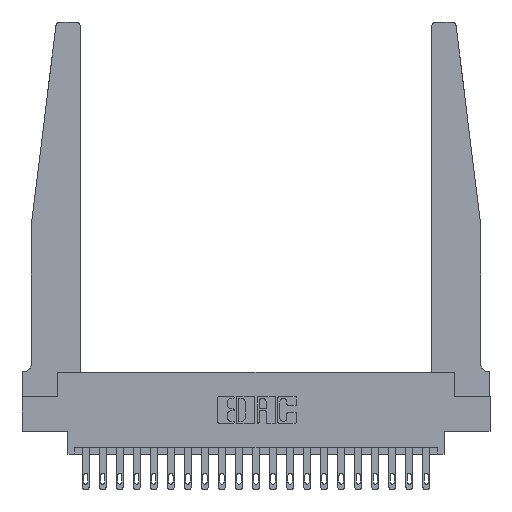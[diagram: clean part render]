
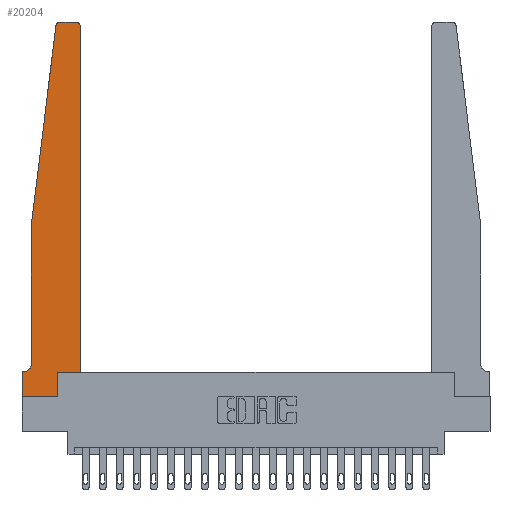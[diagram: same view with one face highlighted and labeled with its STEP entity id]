
A CAD part, top view. The second image highlights one B-rep face of the part: STEP entity #20204.
In plain terms, the highlighted planar face has unit normal (0, 0, 1).
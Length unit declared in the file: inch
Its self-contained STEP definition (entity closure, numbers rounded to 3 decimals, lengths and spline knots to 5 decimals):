
#179 = CARTESIAN_POINT ( 'NONE',  ( 0., 0., 0.37 ) ) ;
#238 = EDGE_CURVE ( 'NONE', #3607, #6068, #4222, .T. ) ;
#278 = CARTESIAN_POINT ( 'NONE',  ( 0.2605, 0.18, 0.37 ) ) ;
#815 = LINE ( 'NONE', #18837, #13661 ) ;
#883 = VECTOR ( 'NONE', #14829, 39.37008 ) ;
#1017 = VECTOR ( 'NONE', #2385, 39.37008 ) ;
#1247 = ORIENTED_EDGE ( 'NONE', *, *, #8335, .T. ) ;
#1311 = CIRCLE ( 'NONE', #14009, 0.05 ) ;
#1351 = LINE ( 'NONE', #5009, #883 ) ;
#1422 = DIRECTION ( 'NONE',  ( 0., 1., 0. ) ) ;
#2039 = ORIENTED_EDGE ( 'NONE', *, *, #21047, .T. ) ;
#2239 = DIRECTION ( 'NONE',  ( 0., 0., -1. ) ) ;
#2385 = DIRECTION ( 'NONE',  ( -1., 0., 0. ) ) ;
#2437 = CARTESIAN_POINT ( 'NONE',  ( 0., 0.1875, 0.37 ) ) ;
#2565 = LINE ( 'NONE', #7774, #5900 ) ;
#2585 = ORIENTED_EDGE ( 'NONE', *, *, #16935, .T. ) ;
#2627 = VECTOR ( 'NONE', #11093, 39.37008 ) ;
#2864 = EDGE_CURVE ( 'NONE', #7976, #3607, #16387, .T. ) ;
#3026 = AXIS2_PLACEMENT_3D ( 'NONE', #9695, #9591, #19854 ) ;
#3241 = CARTESIAN_POINT ( 'NONE',  ( 0.2605, 0., 0.37 ) ) ;
#3318 = CARTESIAN_POINT ( 'NONE',  ( 0.065, 0.2375, 0.37 ) ) ;
#3509 = DIRECTION ( 'NONE',  ( 0., -1., 0. ) ) ;
#3607 = VERTEX_POINT ( 'NONE', #5739 ) ;
#3970 = VERTEX_POINT ( 'NONE', #9327 ) ;
#4222 = LINE ( 'NONE', #18913, #10289 ) ;
#4361 = CARTESIAN_POINT ( 'NONE',  ( 0.27653, 2.75, 0.37 ) ) ;
#4724 = VECTOR ( 'NONE', #3509, 39.37008 ) ;
#5009 = CARTESIAN_POINT ( 'NONE',  ( 0., 0., 0.37 ) ) ;
#5739 = CARTESIAN_POINT ( 'NONE',  ( 0.065, 1.25, 0.37 ) ) ;
#5900 = VECTOR ( 'NONE', #14396, 39.37008 ) ;
#6068 = VERTEX_POINT ( 'NONE', #3318 ) ;
#6510 = AXIS2_PLACEMENT_3D ( 'NONE', #6581, #12978, #16644 ) ;
#6581 = CARTESIAN_POINT ( 'NONE',  ( 0.395, 2.72, 0.37 ) ) ;
#6965 = ORIENTED_EDGE ( 'NONE', *, *, #20962, .T. ) ;
#6979 = LINE ( 'NONE', #13712, #1017 ) ;
#7196 = ORIENTED_EDGE ( 'NONE', *, *, #17585, .T. ) ;
#7213 = DIRECTION ( 'NONE',  ( 0., -1., 0. ) ) ;
#7774 = CARTESIAN_POINT ( 'NONE',  ( 0.2605, 0.18, 0.37 ) ) ;
#7828 = CARTESIAN_POINT ( 'NONE',  ( 0.425, 0.18, 0.37 ) ) ;
#7976 = VERTEX_POINT ( 'NONE', #10484 ) ;
#8082 = CARTESIAN_POINT ( 'NONE',  ( 0.425, 0.18, 0.37 ) ) ;
#8148 = FACE_OUTER_BOUND ( 'NONE', #20293, .T. ) ;
#8335 = EDGE_CURVE ( 'NONE', #17377, #21127, #19267, .T. ) ;
#8602 = CARTESIAN_POINT ( 'NONE',  ( 0.27653, 2.72, 0.37 ) ) ;
#8771 = DIRECTION ( 'NONE',  ( -1., 0., 0. ) ) ;
#9327 = CARTESIAN_POINT ( 'NONE',  ( 0.015, 0.1875, 0.37 ) ) ;
#9474 = PLANE ( 'NONE',  #3026 ) ;
#9478 = VERTEX_POINT ( 'NONE', #16125 ) ;
#9591 = DIRECTION ( 'NONE',  ( 0., 0., 1. ) ) ;
#9695 = CARTESIAN_POINT ( 'NONE',  ( 0., 0.1875, 0.37 ) ) ;
#9772 = EDGE_CURVE ( 'NONE', #11822, #19164, #18864, .T. ) ;
#10076 = ORIENTED_EDGE ( 'NONE', *, *, #10585, .T. ) ;
#10289 = VECTOR ( 'NONE', #7213, 39.37008 ) ;
#10484 = CARTESIAN_POINT ( 'NONE',  ( 0.24675, 2.72367, 0.37 ) ) ;
#10567 = CARTESIAN_POINT ( 'NONE',  ( 0., 0., 0.37 ) ) ;
#10585 = EDGE_CURVE ( 'NONE', #15679, #9478, #13221, .T. ) ;
#10876 = DIRECTION ( 'NONE',  ( -1., 0., 0. ) ) ;
#11093 = DIRECTION ( 'NONE',  ( -0.122, -0.992, 0. ) ) ;
#11538 = CARTESIAN_POINT ( 'NONE',  ( 0.065, 1.25, 0.37 ) ) ;
#11822 = VERTEX_POINT ( 'NONE', #2437 ) ;
#12036 = DIRECTION ( 'NONE',  ( 0., 0., 1. ) ) ;
#12091 = CARTESIAN_POINT ( 'NONE',  ( 0.015, 0.2375, 0.37 ) ) ;
#12157 = EDGE_CURVE ( 'NONE', #3970, #11822, #6979, .T. ) ;
#12176 = ORIENTED_EDGE ( 'NONE', *, *, #17647, .T. ) ;
#12434 = VERTEX_POINT ( 'NONE', #278 ) ;
#12978 = DIRECTION ( 'NONE',  ( 0., 0., 1. ) ) ;
#13125 = CARTESIAN_POINT ( 'NONE',  ( 0.395, 2.75, 0.37 ) ) ;
#13205 = ORIENTED_EDGE ( 'NONE', *, *, #12157, .T. ) ;
#13221 = LINE ( 'NONE', #7828, #21362 ) ;
#13551 = ORIENTED_EDGE ( 'NONE', *, *, #9772, .T. ) ;
#13661 = VECTOR ( 'NONE', #20584, 39.37008 ) ;
#13712 = CARTESIAN_POINT ( 'NONE',  ( 0.065, 0.1875, 0.37 ) ) ;
#13972 = CARTESIAN_POINT ( 'NONE',  ( 0.25, 2.75, 0.37 ) ) ;
#14009 = AXIS2_PLACEMENT_3D ( 'NONE', #12091, #2239, #8771 ) ;
#14396 = DIRECTION ( 'NONE',  ( 0., 1., 0. ) ) ;
#14504 = ORIENTED_EDGE ( 'NONE', *, *, #2864, .T. ) ;
#14829 = DIRECTION ( 'NONE',  ( 1., 0., 0. ) ) ;
#15340 = DIRECTION ( 'NONE',  ( 1., 0., 0. ) ) ;
#15679 = VERTEX_POINT ( 'NONE', #8082 ) ;
#16083 = CIRCLE ( 'NONE', #6510, 0.03 ) ;
#16125 = CARTESIAN_POINT ( 'NONE',  ( 0.425, 2.72, 0.37 ) ) ;
#16387 = LINE ( 'NONE', #11538, #2627 ) ;
#16409 = AXIS2_PLACEMENT_3D ( 'NONE', #8602, #12036, #15340 ) ;
#16482 = VERTEX_POINT ( 'NONE', #3241 ) ;
#16644 = DIRECTION ( 'NONE',  ( 1., 0., 0. ) ) ;
#16935 = EDGE_CURVE ( 'NONE', #19164, #16482, #1351, .T. ) ;
#17377 = VERTEX_POINT ( 'NONE', #13125 ) ;
#17452 = ORIENTED_EDGE ( 'NONE', *, *, #238, .T. ) ;
#17585 = EDGE_CURVE ( 'NONE', #21127, #7976, #20285, .T. ) ;
#17647 = EDGE_CURVE ( 'NONE', #9478, #17377, #16083, .T. ) ;
#18327 = VECTOR ( 'NONE', #10876, 39.37008 ) ;
#18837 = CARTESIAN_POINT ( 'NONE',  ( 0.425, 0.18, 0.37 ) ) ;
#18864 = LINE ( 'NONE', #10567, #4724 ) ;
#18913 = CARTESIAN_POINT ( 'NONE',  ( 0.065, 1.25, 0.37 ) ) ;
#19164 = VERTEX_POINT ( 'NONE', #179 ) ;
#19267 = LINE ( 'NONE', #13972, #18327 ) ;
#19613 = EDGE_CURVE ( 'NONE', #6068, #3970, #1311, .T. ) ;
#19854 = DIRECTION ( 'NONE',  ( 1., 0., 0. ) ) ;
#20204 = ADVANCED_FACE ( 'NONE', ( #8148 ), #9474, .T. ) ;
#20285 = CIRCLE ( 'NONE', #16409, 0.03 ) ;
#20293 = EDGE_LOOP ( 'NONE', ( #1247, #7196, #14504, #17452, #21489, #13205, #13551, #2585, #2039, #6965, #10076, #12176 ) ) ;
#20584 = DIRECTION ( 'NONE',  ( 1., 0., 0. ) ) ;
#20962 = EDGE_CURVE ( 'NONE', #12434, #15679, #815, .T. ) ;
#21047 = EDGE_CURVE ( 'NONE', #16482, #12434, #2565, .T. ) ;
#21127 = VERTEX_POINT ( 'NONE', #4361 ) ;
#21362 = VECTOR ( 'NONE', #1422, 39.37008 ) ;
#21489 = ORIENTED_EDGE ( 'NONE', *, *, #19613, .T. ) ;
